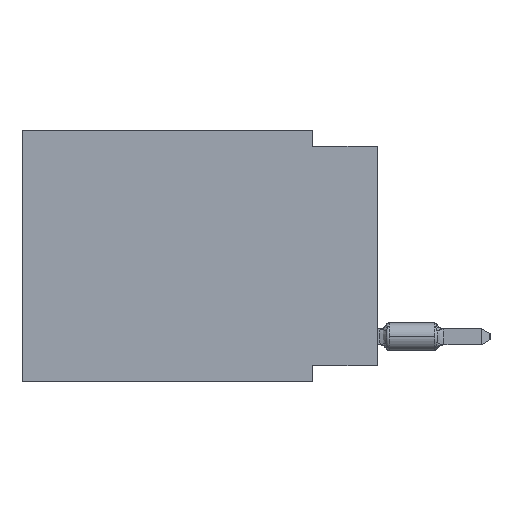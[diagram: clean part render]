
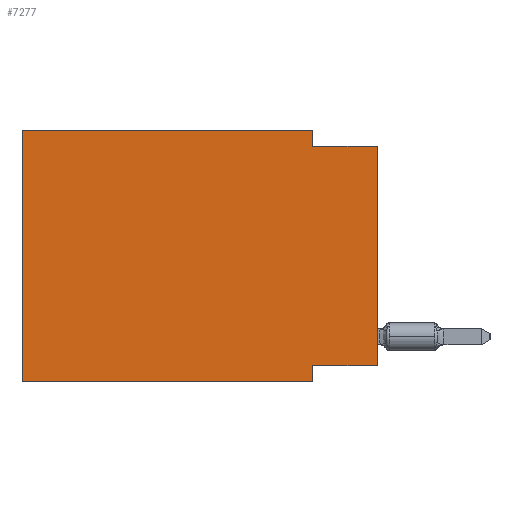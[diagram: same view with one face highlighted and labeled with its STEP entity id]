
A CAD part, left-side view. The second image highlights one B-rep face of the part: STEP entity #7277.
In plain terms, the highlighted planar face has unit normal (-1, 0, 0).
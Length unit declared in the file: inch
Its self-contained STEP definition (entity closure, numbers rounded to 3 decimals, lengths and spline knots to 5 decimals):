
#21 = VECTOR ( 'NONE', #2449, 39.37008 ) ;
#359 = EDGE_CURVE ( 'NONE', #8456, #17366, #20915, .T. ) ;
#630 = CARTESIAN_POINT ( 'NONE',  ( 0., 0.1, -0.39 ) ) ;
#1271 = CARTESIAN_POINT ( 'NONE',  ( 0., 0., -0.365 ) ) ;
#1495 = EDGE_LOOP ( 'NONE', ( #7944, #20734, #21769, #17300, #10622, #10649, #7248, #18871 ) ) ;
#1946 = CARTESIAN_POINT ( 'NONE',  ( 0., 0.1, -0.025 ) ) ;
#2449 = DIRECTION ( 'NONE',  ( 0., -1., 0. ) ) ;
#2657 = DIRECTION ( 'NONE',  ( 0., 0., -1. ) ) ;
#3317 = PLANE ( 'NONE',  #22087 ) ;
#3592 = VECTOR ( 'NONE', #3941, 39.37008 ) ;
#3941 = DIRECTION ( 'NONE',  ( 0., -1., 0. ) ) ;
#3947 = VECTOR ( 'NONE', #4948, 39.37008 ) ;
#4575 = DIRECTION ( 'NONE',  ( 0., 0., -1. ) ) ;
#4616 = VERTEX_POINT ( 'NONE', #7581 ) ;
#4788 = DIRECTION ( 'NONE',  ( 0., 0., -1. ) ) ;
#4948 = DIRECTION ( 'NONE',  ( 0., 0., 1. ) ) ;
#5372 = DIRECTION ( 'NONE',  ( 0., -1., 0. ) ) ;
#5677 = EDGE_CURVE ( 'NONE', #13079, #19338, #13183, .T. ) ;
#6420 = VERTEX_POINT ( 'NONE', #15360 ) ;
#6604 = DIRECTION ( 'NONE',  ( 1., 0., 0. ) ) ;
#7248 = ORIENTED_EDGE ( 'NONE', *, *, #17521, .F. ) ;
#7277 = ADVANCED_FACE ( 'NONE', ( #21880 ), #3317, .F. ) ;
#7581 = CARTESIAN_POINT ( 'NONE',  ( 0., 0.55, -0.39 ) ) ;
#7921 = DIRECTION ( 'NONE',  ( 0., 0., 1. ) ) ;
#7944 = ORIENTED_EDGE ( 'NONE', *, *, #359, .T. ) ;
#8456 = VERTEX_POINT ( 'NONE', #16091 ) ;
#9696 = EDGE_CURVE ( 'NONE', #6420, #13079, #22367, .T. ) ;
#10089 = VECTOR ( 'NONE', #2657, 39.37008 ) ;
#10337 = EDGE_CURVE ( 'NONE', #8456, #13158, #18026, .T. ) ;
#10622 = ORIENTED_EDGE ( 'NONE', *, *, #17913, .F. ) ;
#10649 = ORIENTED_EDGE ( 'NONE', *, *, #18088, .T. ) ;
#10846 = LINE ( 'NONE', #12440, #3592 ) ;
#10937 = CARTESIAN_POINT ( 'NONE',  ( 0., 0., -0.025 ) ) ;
#12440 = CARTESIAN_POINT ( 'NONE',  ( 0., 0.55, -0.39 ) ) ;
#13079 = VERTEX_POINT ( 'NONE', #19075 ) ;
#13158 = VERTEX_POINT ( 'NONE', #16231 ) ;
#13183 = LINE ( 'NONE', #20090, #19502 ) ;
#13303 = VECTOR ( 'NONE', #7921, 39.37008 ) ;
#13672 = CARTESIAN_POINT ( 'NONE',  ( 0., 0., 0. ) ) ;
#15360 = CARTESIAN_POINT ( 'NONE',  ( 0., 0.55, 0. ) ) ;
#15384 = VERTEX_POINT ( 'NONE', #21864 ) ;
#15567 = CARTESIAN_POINT ( 'NONE',  ( 0., 0.55, 0. ) ) ;
#15646 = VECTOR ( 'NONE', #5372, 39.37008 ) ;
#16000 = CARTESIAN_POINT ( 'NONE',  ( 0., 0.55, 0. ) ) ;
#16091 = CARTESIAN_POINT ( 'NONE',  ( 0., 0., -0.365 ) ) ;
#16231 = CARTESIAN_POINT ( 'NONE',  ( 0., 0.1, -0.365 ) ) ;
#16381 = VECTOR ( 'NONE', #19735, 39.37008 ) ;
#16573 = LINE ( 'NONE', #630, #10089 ) ;
#17300 = ORIENTED_EDGE ( 'NONE', *, *, #9696, .F. ) ;
#17366 = VERTEX_POINT ( 'NONE', #18983 ) ;
#17521 = EDGE_CURVE ( 'NONE', #13158, #15384, #16573, .T. ) ;
#17913 = EDGE_CURVE ( 'NONE', #4616, #6420, #21208, .T. ) ;
#18026 = LINE ( 'NONE', #1271, #16381 ) ;
#18088 = EDGE_CURVE ( 'NONE', #4616, #15384, #10846, .T. ) ;
#18871 = ORIENTED_EDGE ( 'NONE', *, *, #10337, .F. ) ;
#18983 = CARTESIAN_POINT ( 'NONE',  ( 0., 0., -0.025 ) ) ;
#19075 = CARTESIAN_POINT ( 'NONE',  ( 0., 0.1, 0. ) ) ;
#19338 = VERTEX_POINT ( 'NONE', #1946 ) ;
#19439 = LINE ( 'NONE', #10937, #21 ) ;
#19502 = VECTOR ( 'NONE', #4575, 39.37008 ) ;
#19735 = DIRECTION ( 'NONE',  ( 0., 1., 0. ) ) ;
#20090 = CARTESIAN_POINT ( 'NONE',  ( 0., 0.1, 0. ) ) ;
#20307 = CARTESIAN_POINT ( 'NONE',  ( 0., 0.55, 0. ) ) ;
#20734 = ORIENTED_EDGE ( 'NONE', *, *, #21097, .F. ) ;
#20915 = LINE ( 'NONE', #13672, #3947 ) ;
#21097 = EDGE_CURVE ( 'NONE', #19338, #17366, #19439, .T. ) ;
#21208 = LINE ( 'NONE', #16000, #13303 ) ;
#21769 = ORIENTED_EDGE ( 'NONE', *, *, #5677, .F. ) ;
#21864 = CARTESIAN_POINT ( 'NONE',  ( 0., 0.1, -0.39 ) ) ;
#21880 = FACE_OUTER_BOUND ( 'NONE', #1495, .T. ) ;
#22087 = AXIS2_PLACEMENT_3D ( 'NONE', #20307, #6604, #4788 ) ;
#22367 = LINE ( 'NONE', #15567, #15646 ) ;
